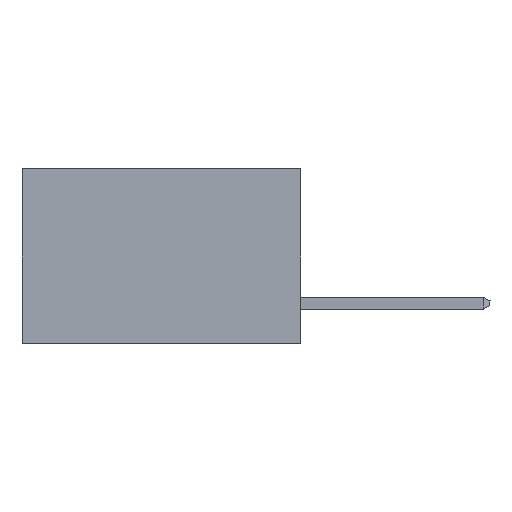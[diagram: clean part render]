
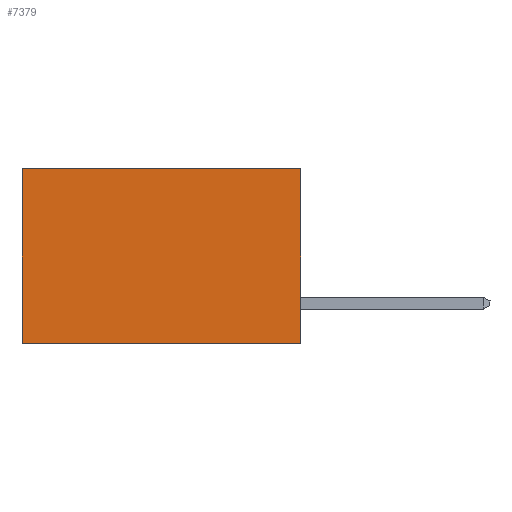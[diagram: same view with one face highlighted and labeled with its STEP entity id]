
A CAD part, left-side view. The second image highlights one B-rep face of the part: STEP entity #7379.
In plain terms, the highlighted planar face has unit normal (-1, 0, 0).
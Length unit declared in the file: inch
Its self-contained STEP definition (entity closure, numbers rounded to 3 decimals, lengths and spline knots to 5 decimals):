
#269 = LINE ( 'NONE', #12017, #12121 ) ;
#839 = DIRECTION ( 'NONE',  ( 0., 1., 0. ) ) ;
#923 = VECTOR ( 'NONE', #7242, 39.37008 ) ;
#1493 = CARTESIAN_POINT ( 'NONE',  ( 0.277, 0.59, -0.37 ) ) ;
#1506 = VECTOR ( 'NONE', #839, 39.37008 ) ;
#1965 = FACE_OUTER_BOUND ( 'NONE', #4958, .T. ) ;
#2424 = CARTESIAN_POINT ( 'NONE',  ( 0.277, 0., -0.37 ) ) ;
#2615 = CARTESIAN_POINT ( 'NONE',  ( 0.277, 0., -0.37 ) ) ;
#3937 = EDGE_CURVE ( 'NONE', #9970, #3954, #269, .T. ) ;
#3954 = VERTEX_POINT ( 'NONE', #7122 ) ;
#4224 = LINE ( 'NONE', #2424, #1506 ) ;
#4459 = VERTEX_POINT ( 'NONE', #2615 ) ;
#4486 = EDGE_CURVE ( 'NONE', #9970, #4459, #5825, .T. ) ;
#4778 = AXIS2_PLACEMENT_3D ( 'NONE', #6007, #5742, #5705 ) ;
#4958 = EDGE_LOOP ( 'NONE', ( #8664, #7405, #9772, #5957 ) ) ;
#5449 = DIRECTION ( 'NONE',  ( 0., 0., -1. ) ) ;
#5705 = DIRECTION ( 'NONE',  ( 0., 0., -1. ) ) ;
#5742 = DIRECTION ( 'NONE',  ( 1., 0., 0. ) ) ;
#5746 = PLANE ( 'NONE',  #4778 ) ;
#5825 = LINE ( 'NONE', #7441, #923 ) ;
#5957 = ORIENTED_EDGE ( 'NONE', *, *, #3937, .T. ) ;
#6007 = CARTESIAN_POINT ( 'NONE',  ( 0.277, 0., -0.37 ) ) ;
#6295 = EDGE_CURVE ( 'NONE', #4459, #9542, #4224, .T. ) ;
#6334 = VECTOR ( 'NONE', #5449, 39.37008 ) ;
#6369 = CARTESIAN_POINT ( 'NONE',  ( 0.277, 0.59, -0.37 ) ) ;
#7020 = CARTESIAN_POINT ( 'NONE',  ( 0.277, 0., 0. ) ) ;
#7122 = CARTESIAN_POINT ( 'NONE',  ( 0.277, 0.59, 0. ) ) ;
#7242 = DIRECTION ( 'NONE',  ( 0., 0., -1. ) ) ;
#7379 = ADVANCED_FACE ( 'NONE', ( #1965 ), #5746, .F. ) ;
#7405 = ORIENTED_EDGE ( 'NONE', *, *, #6295, .F. ) ;
#7441 = CARTESIAN_POINT ( 'NONE',  ( 0.277, 0., -0.37 ) ) ;
#8664 = ORIENTED_EDGE ( 'NONE', *, *, #10166, .T. ) ;
#8758 = LINE ( 'NONE', #1493, #6334 ) ;
#9542 = VERTEX_POINT ( 'NONE', #6369 ) ;
#9772 = ORIENTED_EDGE ( 'NONE', *, *, #4486, .F. ) ;
#9970 = VERTEX_POINT ( 'NONE', #7020 ) ;
#10166 = EDGE_CURVE ( 'NONE', #3954, #9542, #8758, .T. ) ;
#11658 = DIRECTION ( 'NONE',  ( 0., 1., 0. ) ) ;
#12017 = CARTESIAN_POINT ( 'NONE',  ( 0.277, 0., 0. ) ) ;
#12121 = VECTOR ( 'NONE', #11658, 39.37008 ) ;
